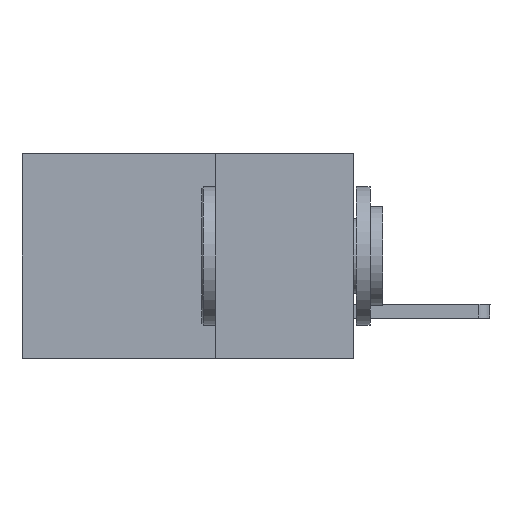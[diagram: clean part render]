
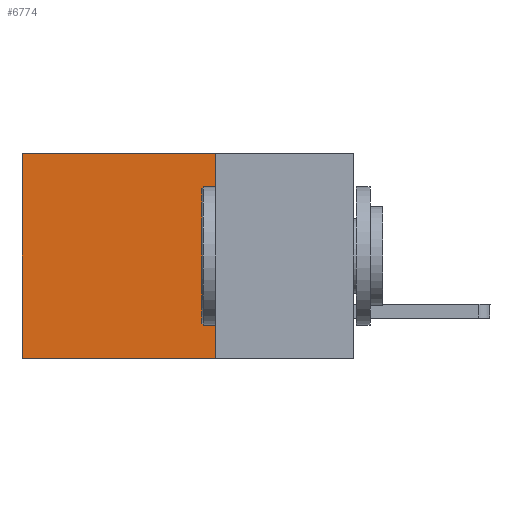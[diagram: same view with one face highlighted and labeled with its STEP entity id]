
A CAD part, left-side view. The second image highlights one B-rep face of the part: STEP entity #6774.
In plain terms, the highlighted planar face has unit normal (-1, 0, 0).
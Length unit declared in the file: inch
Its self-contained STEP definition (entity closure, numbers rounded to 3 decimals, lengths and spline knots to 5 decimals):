
#444 = EDGE_CURVE ( 'NONE', #2851, #5904, #3427, .T. ) ;
#723 = PLANE ( 'NONE',  #1751 ) ;
#1061 = CARTESIAN_POINT ( 'NONE',  ( 0.2875, 0.25, 0. ) ) ;
#1185 = ORIENTED_EDGE ( 'NONE', *, *, #444, .F. ) ;
#1751 = AXIS2_PLACEMENT_3D ( 'NONE', #4028, #7311, #7205 ) ;
#1800 = CARTESIAN_POINT ( 'NONE',  ( 0.2875, 0.6, 0. ) ) ;
#1819 = VECTOR ( 'NONE', #10141, 39.37008 ) ;
#1865 = LINE ( 'NONE', #5241, #8332 ) ;
#2851 = VERTEX_POINT ( 'NONE', #1061 ) ;
#2857 = DIRECTION ( 'NONE',  ( 0., 1., 0. ) ) ;
#3195 = VECTOR ( 'NONE', #4467, 39.37008 ) ;
#3320 = ORIENTED_EDGE ( 'NONE', *, *, #3985, .F. ) ;
#3427 = LINE ( 'NONE', #7726, #9659 ) ;
#3655 = ORIENTED_EDGE ( 'NONE', *, *, #8846, .T. ) ;
#3985 = EDGE_CURVE ( 'NONE', #5904, #7918, #9972, .T. ) ;
#4028 = CARTESIAN_POINT ( 'NONE',  ( 0.2875, 0.25, 0. ) ) ;
#4467 = DIRECTION ( 'NONE',  ( 0., 0., -1. ) ) ;
#5241 = CARTESIAN_POINT ( 'NONE',  ( 0.2875, 0.25, 0. ) ) ;
#5337 = CARTESIAN_POINT ( 'NONE',  ( 0.2875, 0.6, 0. ) ) ;
#5904 = VERTEX_POINT ( 'NONE', #7867 ) ;
#5931 = EDGE_LOOP ( 'NONE', ( #3655, #3320, #1185, #8451 ) ) ;
#6035 = FACE_OUTER_BOUND ( 'NONE', #5931, .T. ) ;
#6487 = EDGE_CURVE ( 'NONE', #2851, #7608, #1865, .T. ) ;
#6774 = ADVANCED_FACE ( 'NONE', ( #6035 ), #723, .F. ) ;
#7205 = DIRECTION ( 'NONE',  ( 0., 0., -1. ) ) ;
#7311 = DIRECTION ( 'NONE',  ( 1., 0., 0. ) ) ;
#7608 = VERTEX_POINT ( 'NONE', #1800 ) ;
#7726 = CARTESIAN_POINT ( 'NONE',  ( 0.2875, 0.25, 0. ) ) ;
#7810 = CARTESIAN_POINT ( 'NONE',  ( 0.2875, 0.25, -0.37 ) ) ;
#7867 = CARTESIAN_POINT ( 'NONE',  ( 0.2875, 0.25, -0.37 ) ) ;
#7918 = VERTEX_POINT ( 'NONE', #10518 ) ;
#8332 = VECTOR ( 'NONE', #2857, 39.37008 ) ;
#8451 = ORIENTED_EDGE ( 'NONE', *, *, #6487, .T. ) ;
#8846 = EDGE_CURVE ( 'NONE', #7608, #7918, #9958, .T. ) ;
#9659 = VECTOR ( 'NONE', #10127, 39.37008 ) ;
#9958 = LINE ( 'NONE', #5337, #3195 ) ;
#9972 = LINE ( 'NONE', #7810, #1819 ) ;
#10127 = DIRECTION ( 'NONE',  ( 0., 0., -1. ) ) ;
#10141 = DIRECTION ( 'NONE',  ( 0., 1., 0. ) ) ;
#10518 = CARTESIAN_POINT ( 'NONE',  ( 0.2875, 0.6, -0.37 ) ) ;
